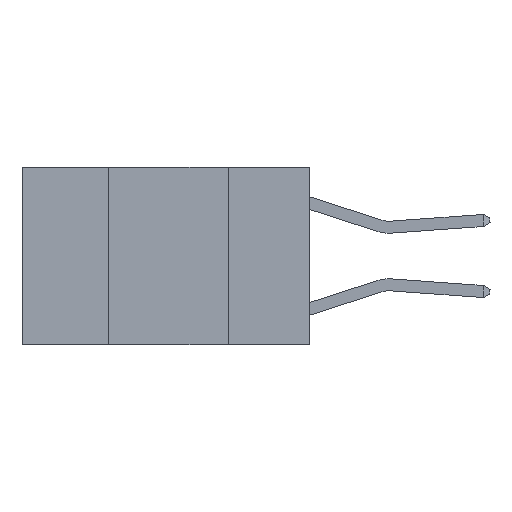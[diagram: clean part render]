
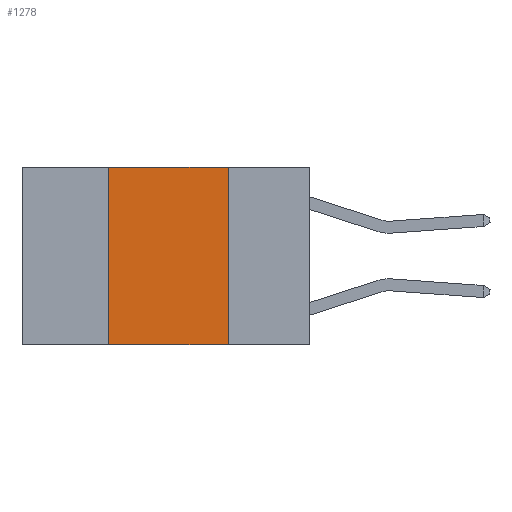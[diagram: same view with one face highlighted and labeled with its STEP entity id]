
A CAD part, left-side view. The second image highlights one B-rep face of the part: STEP entity #1278.
In plain terms, the highlighted planar face has unit normal (-1, 0, 0).
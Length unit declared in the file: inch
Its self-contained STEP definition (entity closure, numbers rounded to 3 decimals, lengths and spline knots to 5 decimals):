
#28 = VERTEX_POINT ( 'NONE', #1373 ) ;
#384 = LINE ( 'NONE', #11107, #4327 ) ;
#1278 = ADVANCED_FACE ( 'NONE', ( #15633 ), #14105, .F. ) ;
#1373 = CARTESIAN_POINT ( 'NONE',  ( 0., 0.17, 0. ) ) ;
#1387 = EDGE_LOOP ( 'NONE', ( #13046, #5682, #11611, #13743 ) ) ;
#2041 = CARTESIAN_POINT ( 'NONE',  ( 0., 0.6, 0. ) ) ;
#3023 = VECTOR ( 'NONE', #8841, 39.37008 ) ;
#3936 = LINE ( 'NONE', #11318, #3023 ) ;
#4327 = VECTOR ( 'NONE', #10060, 39.37008 ) ;
#5431 = CARTESIAN_POINT ( 'NONE',  ( 0., 0.42, 0. ) ) ;
#5600 = CARTESIAN_POINT ( 'NONE',  ( 0., 0.42, 0. ) ) ;
#5682 = ORIENTED_EDGE ( 'NONE', *, *, #8505, .F. ) ;
#8005 = DIRECTION ( 'NONE',  ( 1., 0., 0. ) ) ;
#8505 = EDGE_CURVE ( 'NONE', #15530, #28, #11762, .T. ) ;
#8841 = DIRECTION ( 'NONE',  ( 0., -1., 0. ) ) ;
#9411 = VERTEX_POINT ( 'NONE', #13214 ) ;
#9651 = VECTOR ( 'NONE', #10461, 39.37008 ) ;
#10060 = DIRECTION ( 'NONE',  ( 0., 0., -1. ) ) ;
#10461 = DIRECTION ( 'NONE',  ( 0., -1., 0. ) ) ;
#11107 = CARTESIAN_POINT ( 'NONE',  ( 0., 0.17, 0. ) ) ;
#11221 = VECTOR ( 'NONE', #14011, 39.37008 ) ;
#11318 = CARTESIAN_POINT ( 'NONE',  ( 0., 0.6, -0.37 ) ) ;
#11611 = ORIENTED_EDGE ( 'NONE', *, *, #11675, .F. ) ;
#11675 = EDGE_CURVE ( 'NONE', #9411, #15530, #12882, .T. ) ;
#11762 = LINE ( 'NONE', #11919, #9651 ) ;
#11919 = CARTESIAN_POINT ( 'NONE',  ( 0., 0.6, 0. ) ) ;
#12882 = LINE ( 'NONE', #5431, #11221 ) ;
#12922 = EDGE_CURVE ( 'NONE', #9411, #15790, #3936, .T. ) ;
#13046 = ORIENTED_EDGE ( 'NONE', *, *, #13827, .F. ) ;
#13049 = CARTESIAN_POINT ( 'NONE',  ( 0., 0.17, -0.37 ) ) ;
#13214 = CARTESIAN_POINT ( 'NONE',  ( 0., 0.42, -0.37 ) ) ;
#13743 = ORIENTED_EDGE ( 'NONE', *, *, #12922, .T. ) ;
#13827 = EDGE_CURVE ( 'NONE', #28, #15790, #384, .T. ) ;
#14011 = DIRECTION ( 'NONE',  ( 0., 0., 1. ) ) ;
#14105 = PLANE ( 'NONE',  #14573 ) ;
#14184 = DIRECTION ( 'NONE',  ( 0., 0., -1. ) ) ;
#14573 = AXIS2_PLACEMENT_3D ( 'NONE', #2041, #8005, #14184 ) ;
#15530 = VERTEX_POINT ( 'NONE', #5600 ) ;
#15633 = FACE_OUTER_BOUND ( 'NONE', #1387, .T. ) ;
#15790 = VERTEX_POINT ( 'NONE', #13049 ) ;
